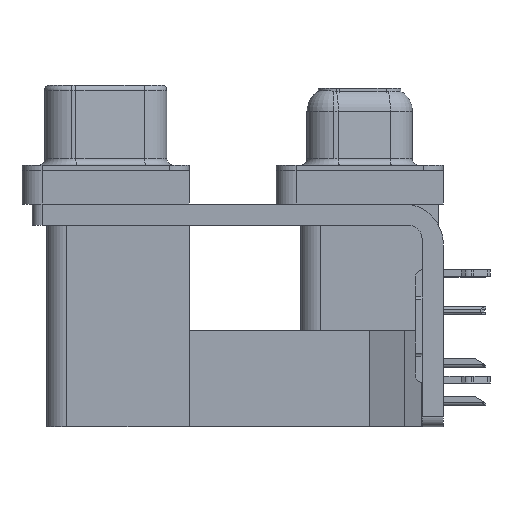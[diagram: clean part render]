
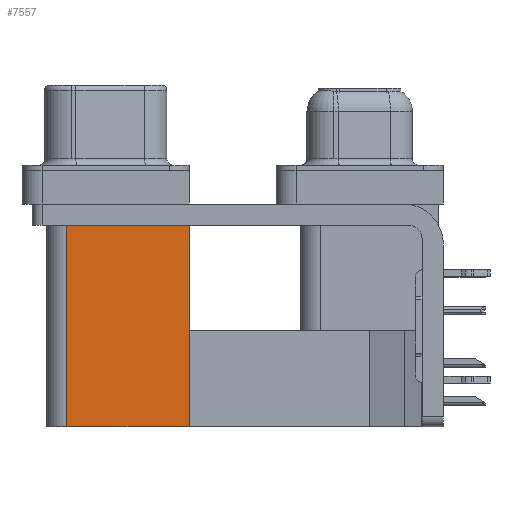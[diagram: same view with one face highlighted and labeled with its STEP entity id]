
A CAD part, left-side view. The second image highlights one B-rep face of the part: STEP entity #7557.
In plain terms, the highlighted planar face has unit normal (-1, 0, 0).
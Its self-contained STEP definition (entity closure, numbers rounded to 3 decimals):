
#51 = LINE ( 'NONE', #33756, #23324 ) ;
#931 = VECTOR ( 'NONE', #25776, 1000. ) ;
#1017 = EDGE_CURVE ( 'NONE', #38398, #16589, #51, .T. ) ;
#1838 = LINE ( 'NONE', #8678, #9976 ) ;
#2466 = VERTEX_POINT ( 'NONE', #35363 ) ;
#2604 = EDGE_CURVE ( 'NONE', #2466, #38398, #1838, .T. ) ;
#3230 = PLANE ( 'NONE',  #20836 ) ;
#5454 = FACE_OUTER_BOUND ( 'NONE', #15568, .T. ) ;
#7557 = ADVANCED_FACE ( 'NONE', ( #5454 ), #3230, .F. ) ;
#8136 = CARTESIAN_POINT ( 'NONE',  ( 3.79, 21.975, -19.2 ) ) ;
#8678 = CARTESIAN_POINT ( 'NONE',  ( 3.79, 12.775, -19.2 ) ) ;
#8902 = CARTESIAN_POINT ( 'NONE',  ( 3.79, 12.775, -19.2 ) ) ;
#9976 = VECTOR ( 'NONE', #29701, 1000. ) ;
#10620 = LINE ( 'NONE', #19910, #931 ) ;
#13378 = ORIENTED_EDGE ( 'NONE', *, *, #1017, .F. ) ;
#13889 = CARTESIAN_POINT ( 'NONE',  ( 3.79, 12.775, -2.5 ) ) ;
#14965 = EDGE_CURVE ( 'NONE', #2466, #39155, #10620, .T. ) ;
#15568 = EDGE_LOOP ( 'NONE', ( #31095, #13378, #18617, #25235 ) ) ;
#15611 = CARTESIAN_POINT ( 'NONE',  ( 3.79, 21.975, -2.5 ) ) ;
#16589 = VERTEX_POINT ( 'NONE', #15611 ) ;
#17758 = DIRECTION ( 'NONE',  ( 1., 0., 0. ) ) ;
#18441 = VECTOR ( 'NONE', #26221, 1000. ) ;
#18617 = ORIENTED_EDGE ( 'NONE', *, *, #2604, .F. ) ;
#19397 = CARTESIAN_POINT ( 'NONE',  ( 3.79, 12.775, -2.5 ) ) ;
#19910 = CARTESIAN_POINT ( 'NONE',  ( 3.79, 12.775, -19.2 ) ) ;
#20347 = EDGE_CURVE ( 'NONE', #39155, #16589, #29458, .T. ) ;
#20836 = AXIS2_PLACEMENT_3D ( 'NONE', #8902, #17758, #37523 ) ;
#21838 = DIRECTION ( 'NONE',  ( 0., 0., 1. ) ) ;
#23324 = VECTOR ( 'NONE', #21838, 1000. ) ;
#25235 = ORIENTED_EDGE ( 'NONE', *, *, #14965, .T. ) ;
#25776 = DIRECTION ( 'NONE',  ( 0., 0., 1. ) ) ;
#26221 = DIRECTION ( 'NONE',  ( 0., 1., 0. ) ) ;
#29458 = LINE ( 'NONE', #13889, #18441 ) ;
#29701 = DIRECTION ( 'NONE',  ( 0., 1., 0. ) ) ;
#31095 = ORIENTED_EDGE ( 'NONE', *, *, #20347, .T. ) ;
#33756 = CARTESIAN_POINT ( 'NONE',  ( 3.79, 21.975, -19.2 ) ) ;
#35363 = CARTESIAN_POINT ( 'NONE',  ( 3.79, 12.775, -19.2 ) ) ;
#37523 = DIRECTION ( 'NONE',  ( 0., 0., -1. ) ) ;
#38398 = VERTEX_POINT ( 'NONE', #8136 ) ;
#39155 = VERTEX_POINT ( 'NONE', #19397 ) ;
